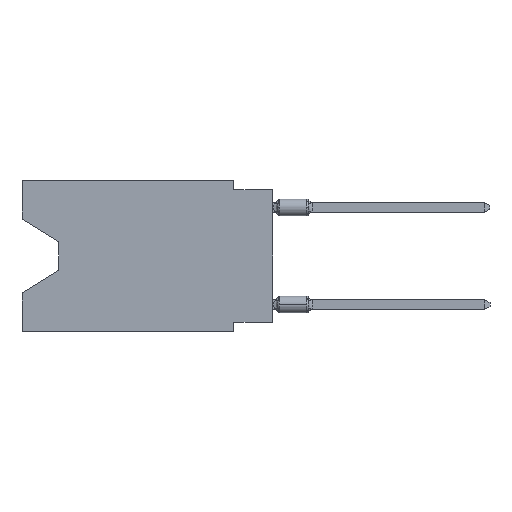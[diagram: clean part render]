
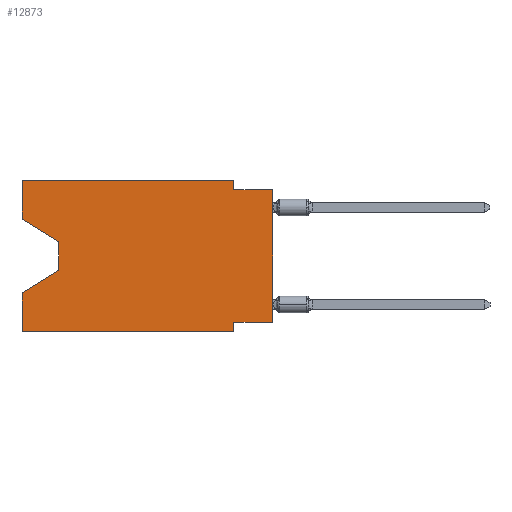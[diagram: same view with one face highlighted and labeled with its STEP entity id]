
A CAD part, left-side view. The second image highlights one B-rep face of the part: STEP entity #12873.
In plain terms, the highlighted planar face has unit normal (-1, 0, 0).
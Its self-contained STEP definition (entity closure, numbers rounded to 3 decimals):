
#21 = VERTEX_POINT ( 'NONE', #5470 ) ;
#116 = LINE ( 'NONE', #6980, #8499 ) ;
#118 = EDGE_CURVE ( 'NONE', #9637, #6758, #3807, .T. ) ;
#308 = EDGE_CURVE ( 'NONE', #9212, #415, #10622, .T. ) ;
#415 = VERTEX_POINT ( 'NONE', #14382 ) ;
#436 = VECTOR ( 'NONE', #10741, 1000. ) ;
#451 = PLANE ( 'NONE',  #7880 ) ;
#845 = LINE ( 'NONE', #4139, #9144 ) ;
#883 = DIRECTION ( 'NONE',  ( 0., -1., 0. ) ) ;
#1093 = DIRECTION ( 'NONE',  ( 0., -1., 0. ) ) ;
#1443 = CARTESIAN_POINT ( 'NONE',  ( 0., 16.383, -7.36 ) ) ;
#1819 = EDGE_CURVE ( 'NONE', #10105, #5174, #845, .T. ) ;
#1925 = VERTEX_POINT ( 'NONE', #7694 ) ;
#2083 = LINE ( 'NONE', #5429, #436 ) ;
#2085 = VERTEX_POINT ( 'NONE', #1443 ) ;
#2444 = LINE ( 'NONE', #6672, #8781 ) ;
#2520 = CARTESIAN_POINT ( 'NONE',  ( 0., 16.383, 0. ) ) ;
#2638 = DIRECTION ( 'NONE',  ( 0., 0., -1. ) ) ;
#2708 = CARTESIAN_POINT ( 'NONE',  ( 0., 2.54, -0.635 ) ) ;
#2772 = DIRECTION ( 'NONE',  ( 0., 0., -1. ) ) ;
#2957 = DIRECTION ( 'NONE',  ( 0., 0., -1. ) ) ;
#3393 = EDGE_CURVE ( 'NONE', #14333, #1925, #2444, .T. ) ;
#3471 = VECTOR ( 'NONE', #10240, 1000. ) ;
#3520 = CARTESIAN_POINT ( 'NONE',  ( 0., 0., 0. ) ) ;
#3524 = FACE_OUTER_BOUND ( 'NONE', #14233, .T. ) ;
#3586 = EDGE_CURVE ( 'NONE', #11328, #10105, #13927, .T. ) ;
#3807 = LINE ( 'NONE', #3520, #12121 ) ;
#3810 = CARTESIAN_POINT ( 'NONE',  ( 0., 16.383, 0. ) ) ;
#3877 = CARTESIAN_POINT ( 'NONE',  ( 0., 2.54, 0. ) ) ;
#4139 = CARTESIAN_POINT ( 'NONE',  ( 0., 2.54, 0. ) ) ;
#4491 = EDGE_CURVE ( 'NONE', #10265, #2085, #2083, .T. ) ;
#4573 = EDGE_CURVE ( 'NONE', #21, #2085, #11399, .T. ) ;
#4651 = CARTESIAN_POINT ( 'NONE',  ( 0., 16.383, 0. ) ) ;
#4710 = CARTESIAN_POINT ( 'NONE',  ( 0., 0., -9.271 ) ) ;
#4822 = DIRECTION ( 'NONE',  ( 0., 0., 1. ) ) ;
#5169 = CARTESIAN_POINT ( 'NONE',  ( 0., 2.54, -9.906 ) ) ;
#5174 = VERTEX_POINT ( 'NONE', #2708 ) ;
#5429 = CARTESIAN_POINT ( 'NONE',  ( 0., 13.97, -5.893 ) ) ;
#5470 = CARTESIAN_POINT ( 'NONE',  ( 0., 16.383, -9.906 ) ) ;
#5503 = DIRECTION ( 'NONE',  ( 0., -0.855, -0.519 ) ) ;
#6239 = ORIENTED_EDGE ( 'NONE', *, *, #11421, .T. ) ;
#6419 = CARTESIAN_POINT ( 'NONE',  ( 0., 0., -0.635 ) ) ;
#6672 = CARTESIAN_POINT ( 'NONE',  ( 0., 16.383, -2.546 ) ) ;
#6720 = VECTOR ( 'NONE', #11908, 1000. ) ;
#6758 = VERTEX_POINT ( 'NONE', #12663 ) ;
#6980 = CARTESIAN_POINT ( 'NONE',  ( 0., 16.383, 0. ) ) ;
#7694 = CARTESIAN_POINT ( 'NONE',  ( 0., 13.97, -4.013 ) ) ;
#7822 = ORIENTED_EDGE ( 'NONE', *, *, #3586, .F. ) ;
#7880 = AXIS2_PLACEMENT_3D ( 'NONE', #3810, #13550, #2638 ) ;
#7938 = LINE ( 'NONE', #12369, #13664 ) ;
#7955 = VECTOR ( 'NONE', #2772, 1000. ) ;
#8046 = EDGE_CURVE ( 'NONE', #14333, #11328, #116, .T. ) ;
#8111 = VECTOR ( 'NONE', #11800, 1000. ) ;
#8248 = CARTESIAN_POINT ( 'NONE',  ( 0., 16.383, -2.546 ) ) ;
#8296 = ORIENTED_EDGE ( 'NONE', *, *, #12021, .T. ) ;
#8450 = CARTESIAN_POINT ( 'NONE',  ( 0., 16.383, 0. ) ) ;
#8499 = VECTOR ( 'NONE', #11404, 1000. ) ;
#8592 = CARTESIAN_POINT ( 'NONE',  ( 0., 13.97, -5.893 ) ) ;
#8665 = EDGE_CURVE ( 'NONE', #5174, #6758, #10713, .T. ) ;
#8690 = ORIENTED_EDGE ( 'NONE', *, *, #8665, .F. ) ;
#8781 = VECTOR ( 'NONE', #5503, 1000. ) ;
#8924 = ORIENTED_EDGE ( 'NONE', *, *, #8046, .F. ) ;
#8984 = ORIENTED_EDGE ( 'NONE', *, *, #4573, .F. ) ;
#9144 = VECTOR ( 'NONE', #2957, 1000. ) ;
#9212 = VERTEX_POINT ( 'NONE', #12276 ) ;
#9622 = ORIENTED_EDGE ( 'NONE', *, *, #4491, .T. ) ;
#9637 = VERTEX_POINT ( 'NONE', #4710 ) ;
#9648 = CARTESIAN_POINT ( 'NONE',  ( 0., 0., -9.271 ) ) ;
#9782 = ORIENTED_EDGE ( 'NONE', *, *, #118, .T. ) ;
#10105 = VERTEX_POINT ( 'NONE', #3877 ) ;
#10240 = DIRECTION ( 'NONE',  ( 0., 0., 1. ) ) ;
#10265 = VERTEX_POINT ( 'NONE', #8592 ) ;
#10622 = LINE ( 'NONE', #5169, #7955 ) ;
#10713 = LINE ( 'NONE', #6419, #14081 ) ;
#10741 = DIRECTION ( 'NONE',  ( 0., 0.855, -0.519 ) ) ;
#10747 = LINE ( 'NONE', #9648, #6720 ) ;
#10770 = ORIENTED_EDGE ( 'NONE', *, *, #308, .F. ) ;
#11328 = VERTEX_POINT ( 'NONE', #8450 ) ;
#11359 = VECTOR ( 'NONE', #1093, 1000. ) ;
#11399 = LINE ( 'NONE', #4651, #3471 ) ;
#11404 = DIRECTION ( 'NONE',  ( 0., 0., 1. ) ) ;
#11421 = EDGE_CURVE ( 'NONE', #21, #415, #13915, .T. ) ;
#11486 = DIRECTION ( 'NONE',  ( 0., 0., -1. ) ) ;
#11768 = ORIENTED_EDGE ( 'NONE', *, *, #12363, .F. ) ;
#11800 = DIRECTION ( 'NONE',  ( 0., -1., 0. ) ) ;
#11908 = DIRECTION ( 'NONE',  ( 0., 1., 0. ) ) ;
#12021 = EDGE_CURVE ( 'NONE', #1925, #10265, #7938, .T. ) ;
#12121 = VECTOR ( 'NONE', #4822, 1000. ) ;
#12276 = CARTESIAN_POINT ( 'NONE',  ( 0., 2.54, -9.271 ) ) ;
#12363 = EDGE_CURVE ( 'NONE', #9637, #9212, #10747, .T. ) ;
#12369 = CARTESIAN_POINT ( 'NONE',  ( 0., 13.97, -4.013 ) ) ;
#12624 = ORIENTED_EDGE ( 'NONE', *, *, #1819, .F. ) ;
#12663 = CARTESIAN_POINT ( 'NONE',  ( 0., 0., -0.635 ) ) ;
#12873 = ADVANCED_FACE ( 'NONE', ( #3524 ), #451, .F. ) ;
#13550 = DIRECTION ( 'NONE',  ( 1., 0., 0. ) ) ;
#13664 = VECTOR ( 'NONE', #11486, 1000. ) ;
#13768 = ORIENTED_EDGE ( 'NONE', *, *, #3393, .T. ) ;
#13915 = LINE ( 'NONE', #14123, #8111 ) ;
#13927 = LINE ( 'NONE', #2520, #11359 ) ;
#14081 = VECTOR ( 'NONE', #883, 1000. ) ;
#14123 = CARTESIAN_POINT ( 'NONE',  ( 0., 16.383, -9.906 ) ) ;
#14233 = EDGE_LOOP ( 'NONE', ( #13768, #8296, #9622, #8984, #6239, #10770, #11768, #9782, #8690, #12624, #7822, #8924 ) ) ;
#14333 = VERTEX_POINT ( 'NONE', #8248 ) ;
#14382 = CARTESIAN_POINT ( 'NONE',  ( 0., 2.54, -9.906 ) ) ;
